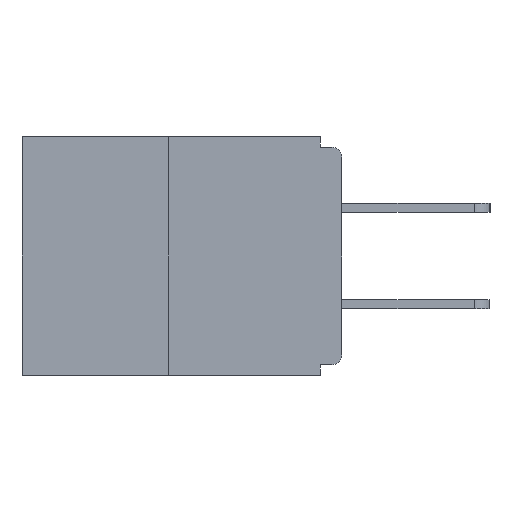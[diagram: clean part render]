
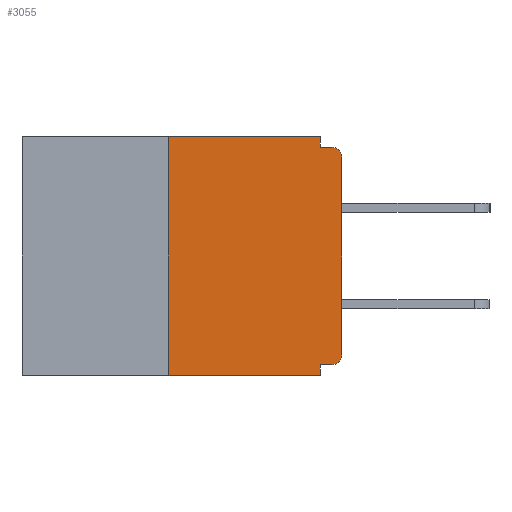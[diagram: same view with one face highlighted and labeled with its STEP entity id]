
A CAD part, left-side view. The second image highlights one B-rep face of the part: STEP entity #3055.
In plain terms, the highlighted planar face has unit normal (-1, 0, 0).
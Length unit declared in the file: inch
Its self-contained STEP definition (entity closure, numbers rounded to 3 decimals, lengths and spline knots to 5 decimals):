
#123 = LINE ( 'NONE', #7648, #7803 ) ;
#320 = EDGE_CURVE ( 'NONE', #352, #8244, #13698, .T. ) ;
#352 = VERTEX_POINT ( 'NONE', #14760 ) ;
#1104 = LINE ( 'NONE', #15108, #15602 ) ;
#1107 = LINE ( 'NONE', #15990, #9470 ) ;
#1157 = DIRECTION ( 'NONE',  ( 0., 0., -1. ) ) ;
#1172 = CARTESIAN_POINT ( 'NONE',  ( 0., 0.25, 0. ) ) ;
#1779 = CIRCLE ( 'NONE', #3070, 0.015 ) ;
#2178 = CARTESIAN_POINT ( 'NONE',  ( 0., 0.015, -0.015 ) ) ;
#2316 = CARTESIAN_POINT ( 'NONE',  ( 0., 0.031, -0.328 ) ) ;
#2598 = CARTESIAN_POINT ( 'NONE',  ( 0., 0., -0.015 ) ) ;
#2702 = ORIENTED_EDGE ( 'NONE', *, *, #320, .F. ) ;
#3055 = ADVANCED_FACE ( 'NONE', ( #15695 ), #4608, .F. ) ;
#3056 = ORIENTED_EDGE ( 'NONE', *, *, #11906, .F. ) ;
#3070 = AXIS2_PLACEMENT_3D ( 'NONE', #4323, #14117, #11700 ) ;
#3396 = VECTOR ( 'NONE', #12491, 39.37008 ) ;
#3467 = CARTESIAN_POINT ( 'NONE',  ( 0., 0., -0.328 ) ) ;
#3726 = VERTEX_POINT ( 'NONE', #4305 ) ;
#3803 = VERTEX_POINT ( 'NONE', #13214 ) ;
#3926 = DIRECTION ( 'NONE',  ( 0., -1., 0. ) ) ;
#4094 = DIRECTION ( 'NONE',  ( 0., -1., 0. ) ) ;
#4200 = CIRCLE ( 'NONE', #11674, 0.015 ) ;
#4224 = AXIS2_PLACEMENT_3D ( 'NONE', #7928, #15378, #4286 ) ;
#4233 = EDGE_LOOP ( 'NONE', ( #8946, #10912, #9796, #5840, #10540, #5117, #9033, #15333, #2702, #3056 ) ) ;
#4286 = DIRECTION ( 'NONE',  ( 0., 0., -1. ) ) ;
#4289 = DIRECTION ( 'NONE',  ( 0., 0., -1. ) ) ;
#4292 = EDGE_CURVE ( 'NONE', #15251, #7786, #4379, .T. ) ;
#4305 = CARTESIAN_POINT ( 'NONE',  ( 0., 0.015, -0.328 ) ) ;
#4323 = CARTESIAN_POINT ( 'NONE',  ( 0., 0.015, -0.03 ) ) ;
#4379 = LINE ( 'NONE', #13282, #14291 ) ;
#4520 = EDGE_CURVE ( 'NONE', #3803, #9873, #10251, .T. ) ;
#4608 = PLANE ( 'NONE',  #4224 ) ;
#5027 = EDGE_CURVE ( 'NONE', #3726, #15251, #7037, .T. ) ;
#5117 = ORIENTED_EDGE ( 'NONE', *, *, #10483, .T. ) ;
#5586 = CARTESIAN_POINT ( 'NONE',  ( 0., 0.031, 0. ) ) ;
#5650 = VERTEX_POINT ( 'NONE', #15556 ) ;
#5840 = ORIENTED_EDGE ( 'NONE', *, *, #4292, .F. ) ;
#6102 = VERTEX_POINT ( 'NONE', #5586 ) ;
#6724 = CARTESIAN_POINT ( 'NONE',  ( 0., 0.015, -0.313 ) ) ;
#7037 = LINE ( 'NONE', #3467, #9498 ) ;
#7648 = CARTESIAN_POINT ( 'NONE',  ( 0., 0.46, -0.343 ) ) ;
#7714 = EDGE_CURVE ( 'NONE', #9873, #6102, #1107, .T. ) ;
#7786 = VERTEX_POINT ( 'NONE', #7899 ) ;
#7803 = VECTOR ( 'NONE', #3926, 39.37008 ) ;
#7899 = CARTESIAN_POINT ( 'NONE',  ( 0., 0.031, -0.343 ) ) ;
#7928 = CARTESIAN_POINT ( 'NONE',  ( 0., 0.46, 0. ) ) ;
#8015 = DIRECTION ( 'NONE',  ( 0., 0., -1. ) ) ;
#8244 = VERTEX_POINT ( 'NONE', #2178 ) ;
#8946 = ORIENTED_EDGE ( 'NONE', *, *, #7714, .F. ) ;
#9033 = ORIENTED_EDGE ( 'NONE', *, *, #12858, .T. ) ;
#9050 = CARTESIAN_POINT ( 'NONE',  ( 0., 0.25, 0. ) ) ;
#9470 = VECTOR ( 'NONE', #4094, 39.37008 ) ;
#9498 = VECTOR ( 'NONE', #13038, 39.37008 ) ;
#9796 = ORIENTED_EDGE ( 'NONE', *, *, #11725, .T. ) ;
#9873 = VERTEX_POINT ( 'NONE', #1172 ) ;
#10175 = DIRECTION ( 'NONE',  ( 0., 0., 1. ) ) ;
#10223 = EDGE_CURVE ( 'NONE', #11039, #8244, #1779, .T. ) ;
#10251 = LINE ( 'NONE', #9050, #13620 ) ;
#10483 = EDGE_CURVE ( 'NONE', #3726, #5650, #4200, .T. ) ;
#10540 = ORIENTED_EDGE ( 'NONE', *, *, #5027, .F. ) ;
#10713 = LINE ( 'NONE', #13235, #13255 ) ;
#10749 = CARTESIAN_POINT ( 'NONE',  ( 0., 0., -0.03 ) ) ;
#10912 = ORIENTED_EDGE ( 'NONE', *, *, #4520, .F. ) ;
#11039 = VERTEX_POINT ( 'NONE', #10749 ) ;
#11493 = DIRECTION ( 'NONE',  ( -1., 0., 0. ) ) ;
#11674 = AXIS2_PLACEMENT_3D ( 'NONE', #6724, #11493, #8015 ) ;
#11700 = DIRECTION ( 'NONE',  ( 0., 0., -1. ) ) ;
#11725 = EDGE_CURVE ( 'NONE', #3803, #7786, #123, .T. ) ;
#11906 = EDGE_CURVE ( 'NONE', #6102, #352, #10713, .T. ) ;
#12491 = DIRECTION ( 'NONE',  ( 0., -1., 0. ) ) ;
#12858 = EDGE_CURVE ( 'NONE', #5650, #11039, #1104, .T. ) ;
#13038 = DIRECTION ( 'NONE',  ( 0., 1., 0. ) ) ;
#13214 = CARTESIAN_POINT ( 'NONE',  ( 0., 0.25, -0.343 ) ) ;
#13235 = CARTESIAN_POINT ( 'NONE',  ( 0., 0.031, 0. ) ) ;
#13255 = VECTOR ( 'NONE', #1157, 39.37008 ) ;
#13282 = CARTESIAN_POINT ( 'NONE',  ( 0., 0.031, -0.343 ) ) ;
#13620 = VECTOR ( 'NONE', #10175, 39.37008 ) ;
#13698 = LINE ( 'NONE', #2598, #3396 ) ;
#13725 = DIRECTION ( 'NONE',  ( 0., 0., 1. ) ) ;
#14117 = DIRECTION ( 'NONE',  ( -1., 0., 0. ) ) ;
#14291 = VECTOR ( 'NONE', #4289, 39.37008 ) ;
#14760 = CARTESIAN_POINT ( 'NONE',  ( 0., 0.031, -0.015 ) ) ;
#15108 = CARTESIAN_POINT ( 'NONE',  ( 0., 0., 0. ) ) ;
#15251 = VERTEX_POINT ( 'NONE', #2316 ) ;
#15333 = ORIENTED_EDGE ( 'NONE', *, *, #10223, .T. ) ;
#15378 = DIRECTION ( 'NONE',  ( 1., 0., 0. ) ) ;
#15556 = CARTESIAN_POINT ( 'NONE',  ( 0., 0., -0.313 ) ) ;
#15602 = VECTOR ( 'NONE', #13725, 39.37008 ) ;
#15695 = FACE_OUTER_BOUND ( 'NONE', #4233, .T. ) ;
#15990 = CARTESIAN_POINT ( 'NONE',  ( 0., 0.46, 0. ) ) ;
